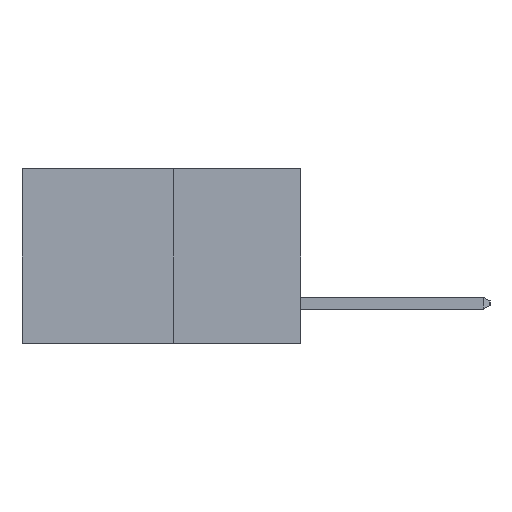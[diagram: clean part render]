
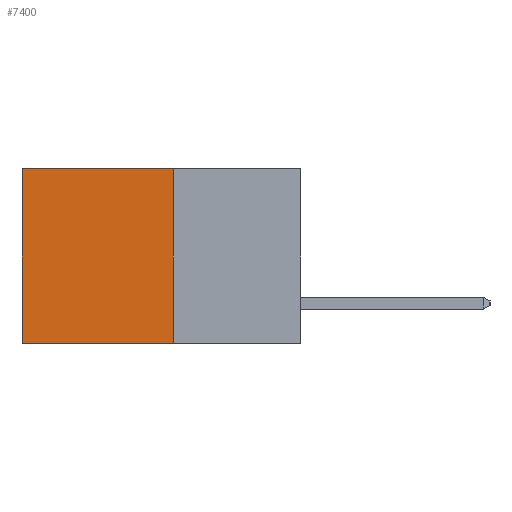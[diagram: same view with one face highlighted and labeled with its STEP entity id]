
A CAD part, left-side view. The second image highlights one B-rep face of the part: STEP entity #7400.
In plain terms, the highlighted planar face has unit normal (-1, 0, 0).
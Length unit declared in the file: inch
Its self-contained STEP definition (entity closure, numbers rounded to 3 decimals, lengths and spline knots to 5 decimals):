
#2 = VERTEX_POINT ( 'NONE', #13088 ) ;
#1000 = DIRECTION ( 'NONE',  ( 0., 0., -1. ) ) ;
#2730 = EDGE_CURVE ( 'NONE', #11460, #10511, #16998, .T. ) ;
#2969 = ORIENTED_EDGE ( 'NONE', *, *, #5501, .F. ) ;
#3023 = CARTESIAN_POINT ( 'NONE',  ( 0.277, 0.27, -0.37 ) ) ;
#5088 = DIRECTION ( 'NONE',  ( 0., 0., -1. ) ) ;
#5160 = EDGE_CURVE ( 'NONE', #10511, #22757, #22196, .T. ) ;
#5501 = EDGE_CURVE ( 'NONE', #11460, #2, #20128, .T. ) ;
#5920 = CARTESIAN_POINT ( 'NONE',  ( 0.277, 0.59, -0.37 ) ) ;
#6853 = VECTOR ( 'NONE', #13674, 39.37008 ) ;
#7400 = ADVANCED_FACE ( 'NONE', ( #12936 ), #10944, .F. ) ;
#8297 = CARTESIAN_POINT ( 'NONE',  ( 0.277, 0.59, 0. ) ) ;
#9009 = VECTOR ( 'NONE', #14779, 39.37008 ) ;
#10511 = VERTEX_POINT ( 'NONE', #8297 ) ;
#10670 = ORIENTED_EDGE ( 'NONE', *, *, #2730, .T. ) ;
#10944 = PLANE ( 'NONE',  #15668 ) ;
#11460 = VERTEX_POINT ( 'NONE', #20538 ) ;
#12233 = EDGE_LOOP ( 'NONE', ( #23654, #21286, #2969, #10670 ) ) ;
#12816 = CARTESIAN_POINT ( 'NONE',  ( 0.277, 0.27, -0.37 ) ) ;
#12936 = FACE_OUTER_BOUND ( 'NONE', #12233, .T. ) ;
#13088 = CARTESIAN_POINT ( 'NONE',  ( 0.277, 0.27, -0.37 ) ) ;
#13674 = DIRECTION ( 'NONE',  ( 0., 0., -1. ) ) ;
#14441 = VECTOR ( 'NONE', #1000, 39.37008 ) ;
#14779 = DIRECTION ( 'NONE',  ( 0., 1., 0. ) ) ;
#14922 = CARTESIAN_POINT ( 'NONE',  ( 0.277, 0.27, -0.37 ) ) ;
#15668 = AXIS2_PLACEMENT_3D ( 'NONE', #3023, #16772, #5088 ) ;
#16166 = CARTESIAN_POINT ( 'NONE',  ( 0.277, 0.27, 0. ) ) ;
#16772 = DIRECTION ( 'NONE',  ( 1., 0., 0. ) ) ;
#16998 = LINE ( 'NONE', #16166, #22028 ) ;
#19996 = DIRECTION ( 'NONE',  ( 0., 1., 0. ) ) ;
#20128 = LINE ( 'NONE', #14922, #14441 ) ;
#20433 = EDGE_CURVE ( 'NONE', #2, #22757, #23692, .T. ) ;
#20538 = CARTESIAN_POINT ( 'NONE',  ( 0.277, 0.27, 0. ) ) ;
#21181 = CARTESIAN_POINT ( 'NONE',  ( 0.277, 0.59, -0.37 ) ) ;
#21286 = ORIENTED_EDGE ( 'NONE', *, *, #20433, .F. ) ;
#22028 = VECTOR ( 'NONE', #19996, 39.37008 ) ;
#22196 = LINE ( 'NONE', #5920, #6853 ) ;
#22757 = VERTEX_POINT ( 'NONE', #21181 ) ;
#23654 = ORIENTED_EDGE ( 'NONE', *, *, #5160, .T. ) ;
#23692 = LINE ( 'NONE', #12816, #9009 ) ;
